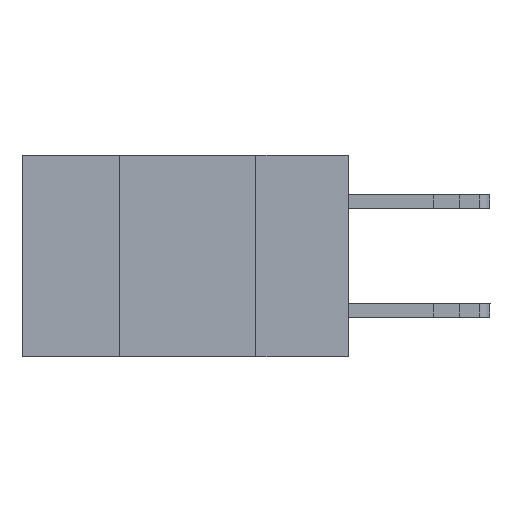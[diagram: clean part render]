
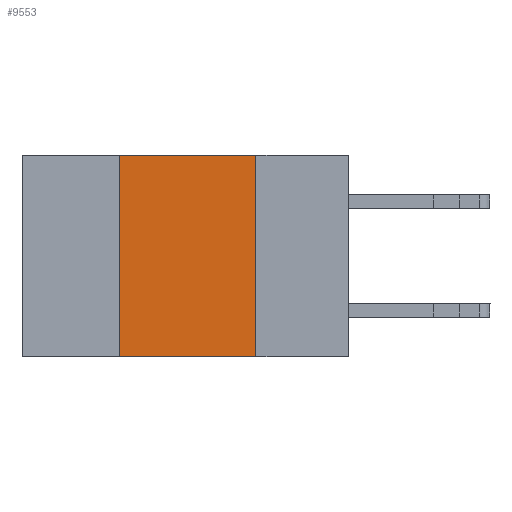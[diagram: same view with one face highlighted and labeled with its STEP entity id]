
A CAD part, left-side view. The second image highlights one B-rep face of the part: STEP entity #9553.
In plain terms, the highlighted planar face has unit normal (-1, 0, 0).
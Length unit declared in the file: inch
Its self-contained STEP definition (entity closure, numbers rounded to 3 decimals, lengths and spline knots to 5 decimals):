
#184 = VERTEX_POINT ( 'NONE', #10836 ) ;
#779 = CARTESIAN_POINT ( 'NONE',  ( 0., 0.17, 0. ) ) ;
#795 = ORIENTED_EDGE ( 'NONE', *, *, #10578, .F. ) ;
#1444 = EDGE_CURVE ( 'NONE', #5768, #184, #11606, .T. ) ;
#1482 = DIRECTION ( 'NONE',  ( 0., -1., 0. ) ) ;
#1521 = ORIENTED_EDGE ( 'NONE', *, *, #1444, .F. ) ;
#2956 = CARTESIAN_POINT ( 'NONE',  ( 0., 0.6, 0. ) ) ;
#3910 = CARTESIAN_POINT ( 'NONE',  ( 0., 0.42, 0. ) ) ;
#4105 = VECTOR ( 'NONE', #13362, 39.37008 ) ;
#4133 = DIRECTION ( 'NONE',  ( 1., 0., 0. ) ) ;
#4263 = LINE ( 'NONE', #12146, #4105 ) ;
#4665 = FACE_OUTER_BOUND ( 'NONE', #5405, .T. ) ;
#5405 = EDGE_LOOP ( 'NONE', ( #1521, #12458, #795, #7847 ) ) ;
#5553 = VECTOR ( 'NONE', #8364, 39.37008 ) ;
#5768 = VERTEX_POINT ( 'NONE', #779 ) ;
#6909 = EDGE_CURVE ( 'NONE', #10135, #184, #4263, .T. ) ;
#7115 = CARTESIAN_POINT ( 'NONE',  ( 0., 0.42, -0.37 ) ) ;
#7388 = DIRECTION ( 'NONE',  ( 0., 0., -1. ) ) ;
#7709 = AXIS2_PLACEMENT_3D ( 'NONE', #2956, #4133, #7388 ) ;
#7760 = VECTOR ( 'NONE', #1482, 39.37008 ) ;
#7847 = ORIENTED_EDGE ( 'NONE', *, *, #6909, .T. ) ;
#7902 = DIRECTION ( 'NONE',  ( 0., 0., 1. ) ) ;
#8347 = LINE ( 'NONE', #12102, #7760 ) ;
#8364 = DIRECTION ( 'NONE',  ( 0., 0., -1. ) ) ;
#8560 = CARTESIAN_POINT ( 'NONE',  ( 0., 0.17, 0. ) ) ;
#8996 = CARTESIAN_POINT ( 'NONE',  ( 0., 0.42, 0. ) ) ;
#9553 = ADVANCED_FACE ( 'NONE', ( #4665 ), #10569, .F. ) ;
#10135 = VERTEX_POINT ( 'NONE', #7115 ) ;
#10569 = PLANE ( 'NONE',  #7709 ) ;
#10578 = EDGE_CURVE ( 'NONE', #10135, #11569, #11051, .T. ) ;
#10836 = CARTESIAN_POINT ( 'NONE',  ( 0., 0.17, -0.37 ) ) ;
#11051 = LINE ( 'NONE', #8996, #12910 ) ;
#11569 = VERTEX_POINT ( 'NONE', #3910 ) ;
#11606 = LINE ( 'NONE', #8560, #5553 ) ;
#11960 = EDGE_CURVE ( 'NONE', #11569, #5768, #8347, .T. ) ;
#12102 = CARTESIAN_POINT ( 'NONE',  ( 0., 0.6, 0. ) ) ;
#12146 = CARTESIAN_POINT ( 'NONE',  ( 0., 0.6, -0.37 ) ) ;
#12458 = ORIENTED_EDGE ( 'NONE', *, *, #11960, .F. ) ;
#12910 = VECTOR ( 'NONE', #7902, 39.37008 ) ;
#13362 = DIRECTION ( 'NONE',  ( 0., -1., 0. ) ) ;
